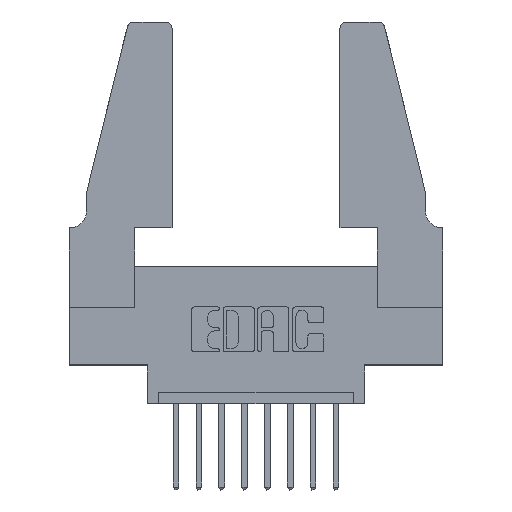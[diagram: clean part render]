
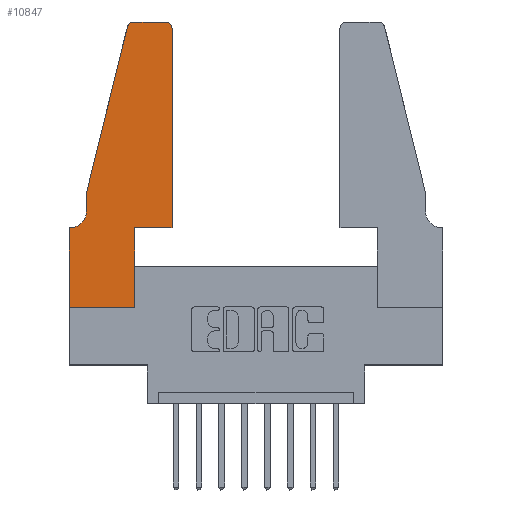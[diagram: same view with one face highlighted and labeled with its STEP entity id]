
A CAD part, top view. The second image highlights one B-rep face of the part: STEP entity #10847.
In plain terms, the highlighted planar face has unit normal (0, 0, 1).
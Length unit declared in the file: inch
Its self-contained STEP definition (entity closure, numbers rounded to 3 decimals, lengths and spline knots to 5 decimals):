
#14 = ORIENTED_EDGE ( 'NONE', *, *, #1918, .T. ) ;
#96 = VECTOR ( 'NONE', #9102, 39.37008 ) ;
#185 = CARTESIAN_POINT ( 'NONE',  ( 0.0055, 0.42, 0.37 ) ) ;
#402 = DIRECTION ( 'NONE',  ( 0., -1., 0. ) ) ;
#431 = AXIS2_PLACEMENT_3D ( 'NONE', #185, #6203, #1211 ) ;
#468 = EDGE_CURVE ( 'NONE', #724, #8885, #2731, .T. ) ;
#702 = DIRECTION ( 'NONE',  ( -1., 0., 0. ) ) ;
#724 = VERTEX_POINT ( 'NONE', #2084 ) ;
#790 = CARTESIAN_POINT ( 'NONE',  ( 0.2865, 0.35, 0.37 ) ) ;
#793 = PLANE ( 'NONE',  #5079 ) ;
#859 = LINE ( 'NONE', #3029, #96 ) ;
#886 = CARTESIAN_POINT ( 'NONE',  ( 0.4505, 0.35, 0.37 ) ) ;
#947 = LINE ( 'NONE', #5987, #6109 ) ;
#1071 = CIRCLE ( 'NONE', #12181, 0.03 ) ;
#1192 = VERTEX_POINT ( 'NONE', #3799 ) ;
#1211 = DIRECTION ( 'NONE',  ( -1., 0., 0. ) ) ;
#1384 = EDGE_CURVE ( 'NONE', #8885, #3853, #859, .T. ) ;
#1406 = ORIENTED_EDGE ( 'NONE', *, *, #4951, .T. ) ;
#1485 = ORIENTED_EDGE ( 'NONE', *, *, #1384, .T. ) ;
#1540 = CARTESIAN_POINT ( 'NONE',  ( 0.284, 1.22, 0.37 ) ) ;
#1575 = CARTESIAN_POINT ( 'NONE',  ( 0.0755, 0.42, 0.37 ) ) ;
#1616 = DIRECTION ( 'NONE',  ( 1., 0., 0. ) ) ;
#1655 = CARTESIAN_POINT ( 'NONE',  ( 0.0755, 0.5, 0.37 ) ) ;
#1918 = EDGE_CURVE ( 'NONE', #3746, #5044, #9951, .T. ) ;
#2084 = CARTESIAN_POINT ( 'NONE',  ( 0.284, 1.25, 0.37 ) ) ;
#2662 = EDGE_CURVE ( 'NONE', #11265, #1192, #6472, .T. ) ;
#2731 = CIRCLE ( 'NONE', #8522, 0.03 ) ;
#2782 = CARTESIAN_POINT ( 'NONE',  ( 0.0755, 0.35, 0.37 ) ) ;
#3029 = CARTESIAN_POINT ( 'NONE',  ( 0.0755, 0.5, 0.37 ) ) ;
#3341 = CARTESIAN_POINT ( 'NONE',  ( 0.25487, 1.22718, 0.37 ) ) ;
#3538 = ORIENTED_EDGE ( 'NONE', *, *, #4071, .T. ) ;
#3583 = ORIENTED_EDGE ( 'NONE', *, *, #5537, .T. ) ;
#3612 = CIRCLE ( 'NONE', #431, 0.07 ) ;
#3746 = VERTEX_POINT ( 'NONE', #5218 ) ;
#3799 = CARTESIAN_POINT ( 'NONE',  ( 0.2865, 0.35, 0.37 ) ) ;
#3853 = VERTEX_POINT ( 'NONE', #1655 ) ;
#4071 = EDGE_CURVE ( 'NONE', #12822, #3746, #3612, .T. ) ;
#4336 = EDGE_CURVE ( 'NONE', #1192, #6003, #10066, .T. ) ;
#4497 = CARTESIAN_POINT ( 'NONE',  ( 0.2605, 1.25, 0.37 ) ) ;
#4536 = VECTOR ( 'NONE', #11347, 39.37008 ) ;
#4542 = EDGE_LOOP ( 'NONE', ( #10383, #8750, #1485, #1406, #3538, #14, #10300, #11840, #5856, #10246, #12100, #3583 ) ) ;
#4595 = VECTOR ( 'NONE', #6889, 39.37008 ) ;
#4765 = DIRECTION ( 'NONE',  ( 0., 1., 0. ) ) ;
#4921 = VERTEX_POINT ( 'NONE', #12155 ) ;
#4951 = EDGE_CURVE ( 'NONE', #3853, #12822, #9420, .T. ) ;
#5044 = VERTEX_POINT ( 'NONE', #8575 ) ;
#5079 = AXIS2_PLACEMENT_3D ( 'NONE', #9913, #11862, #11902 ) ;
#5218 = CARTESIAN_POINT ( 'NONE',  ( 0.0055, 0.35, 0.37 ) ) ;
#5537 = EDGE_CURVE ( 'NONE', #10205, #4921, #1071, .T. ) ;
#5589 = DIRECTION ( 'NONE',  ( 1., 0., 0. ) ) ;
#5786 = LINE ( 'NONE', #8517, #9255 ) ;
#5856 = ORIENTED_EDGE ( 'NONE', *, *, #2662, .T. ) ;
#5987 = CARTESIAN_POINT ( 'NONE',  ( 0., 0., 0.37 ) ) ;
#6003 = VERTEX_POINT ( 'NONE', #886 ) ;
#6109 = VECTOR ( 'NONE', #6968, 39.37008 ) ;
#6203 = DIRECTION ( 'NONE',  ( 0., 0., -1. ) ) ;
#6315 = VECTOR ( 'NONE', #702, 39.37008 ) ;
#6472 = LINE ( 'NONE', #790, #11514 ) ;
#6746 = VECTOR ( 'NONE', #1616, 39.37008 ) ;
#6889 = DIRECTION ( 'NONE',  ( 0., 1., 0. ) ) ;
#6942 = LINE ( 'NONE', #10867, #4595 ) ;
#6968 = DIRECTION ( 'NONE',  ( 1., 0., 0. ) ) ;
#7061 = CARTESIAN_POINT ( 'NONE',  ( 0.4505, 1.22, 0.37 ) ) ;
#7103 = CARTESIAN_POINT ( 'NONE',  ( 0.2865, 0., 0.37 ) ) ;
#7588 = DIRECTION ( 'NONE',  ( 1., 0., 0. ) ) ;
#7930 = LINE ( 'NONE', #4497, #8402 ) ;
#8202 = EDGE_CURVE ( 'NONE', #4921, #724, #7930, .T. ) ;
#8325 = CARTESIAN_POINT ( 'NONE',  ( 0., 0., 0.37 ) ) ;
#8402 = VECTOR ( 'NONE', #8587, 39.37008 ) ;
#8517 = CARTESIAN_POINT ( 'NONE',  ( 0., 0., 0.37 ) ) ;
#8522 = AXIS2_PLACEMENT_3D ( 'NONE', #1540, #8668, #5589 ) ;
#8574 = CARTESIAN_POINT ( 'NONE',  ( 0.4205, 1.22, 0.37 ) ) ;
#8575 = CARTESIAN_POINT ( 'NONE',  ( 0., 0.35, 0.37 ) ) ;
#8587 = DIRECTION ( 'NONE',  ( -1., 0., 0. ) ) ;
#8668 = DIRECTION ( 'NONE',  ( 0., 0., 1. ) ) ;
#8750 = ORIENTED_EDGE ( 'NONE', *, *, #468, .T. ) ;
#8885 = VERTEX_POINT ( 'NONE', #3341 ) ;
#8996 = EDGE_CURVE ( 'NONE', #6003, #10205, #6942, .T. ) ;
#9102 = DIRECTION ( 'NONE',  ( -0.239, -0.971, 0. ) ) ;
#9128 = FACE_OUTER_BOUND ( 'NONE', #4542, .T. ) ;
#9199 = VERTEX_POINT ( 'NONE', #8325 ) ;
#9255 = VECTOR ( 'NONE', #402, 39.37008 ) ;
#9420 = LINE ( 'NONE', #12200, #4536 ) ;
#9541 = CARTESIAN_POINT ( 'NONE',  ( 0.4505, 0.35, 0.37 ) ) ;
#9595 = DIRECTION ( 'NONE',  ( 0., 0., 1. ) ) ;
#9913 = CARTESIAN_POINT ( 'NONE',  ( 0., 0.35, 0.37 ) ) ;
#9951 = LINE ( 'NONE', #2782, #6315 ) ;
#10066 = LINE ( 'NONE', #9541, #6746 ) ;
#10205 = VERTEX_POINT ( 'NONE', #7061 ) ;
#10246 = ORIENTED_EDGE ( 'NONE', *, *, #4336, .T. ) ;
#10300 = ORIENTED_EDGE ( 'NONE', *, *, #12759, .T. ) ;
#10383 = ORIENTED_EDGE ( 'NONE', *, *, #8202, .T. ) ;
#10847 = ADVANCED_FACE ( 'NONE', ( #9128 ), #793, .T. ) ;
#10867 = CARTESIAN_POINT ( 'NONE',  ( 0.4505, 0.35, 0.37 ) ) ;
#11265 = VERTEX_POINT ( 'NONE', #7103 ) ;
#11277 = EDGE_CURVE ( 'NONE', #9199, #11265, #947, .T. ) ;
#11347 = DIRECTION ( 'NONE',  ( 0., -1., 0. ) ) ;
#11514 = VECTOR ( 'NONE', #4765, 39.37008 ) ;
#11840 = ORIENTED_EDGE ( 'NONE', *, *, #11277, .T. ) ;
#11862 = DIRECTION ( 'NONE',  ( 0., 0., 1. ) ) ;
#11902 = DIRECTION ( 'NONE',  ( 1., 0., 0. ) ) ;
#12100 = ORIENTED_EDGE ( 'NONE', *, *, #8996, .T. ) ;
#12155 = CARTESIAN_POINT ( 'NONE',  ( 0.4205, 1.25, 0.37 ) ) ;
#12181 = AXIS2_PLACEMENT_3D ( 'NONE', #8574, #9595, #7588 ) ;
#12200 = CARTESIAN_POINT ( 'NONE',  ( 0.0755, 0.5, 0.37 ) ) ;
#12759 = EDGE_CURVE ( 'NONE', #5044, #9199, #5786, .T. ) ;
#12822 = VERTEX_POINT ( 'NONE', #1575 ) ;
